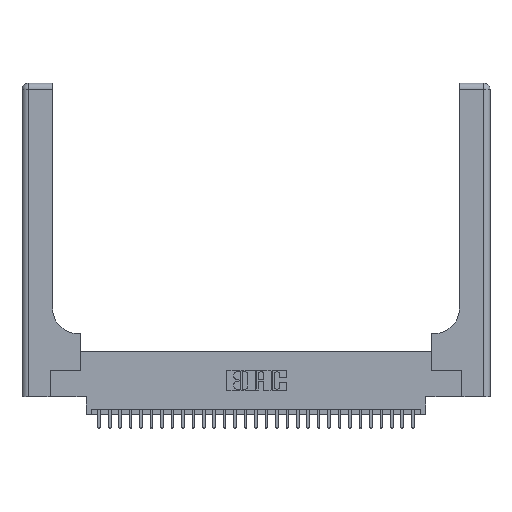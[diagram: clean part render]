
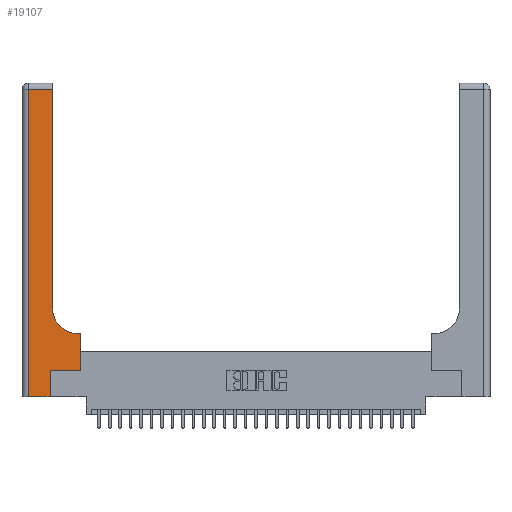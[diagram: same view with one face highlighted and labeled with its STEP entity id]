
A CAD part, top view. The second image highlights one B-rep face of the part: STEP entity #19107.
In plain terms, the highlighted planar face has unit normal (0, 0, 1).
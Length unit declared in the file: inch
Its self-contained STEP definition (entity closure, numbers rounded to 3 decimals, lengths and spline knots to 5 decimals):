
#305 = ORIENTED_EDGE ( 'NONE', *, *, #15811, .T. ) ;
#684 = VECTOR ( 'NONE', #5608, 39.37008 ) ;
#1043 = VERTEX_POINT ( 'NONE', #20322 ) ;
#1319 = DIRECTION ( 'NONE',  ( 1., 0., 0. ) ) ;
#2099 = EDGE_CURVE ( 'NONE', #4533, #7170, #13549, .T. ) ;
#2266 = ORIENTED_EDGE ( 'NONE', *, *, #24593, .T. ) ;
#2350 = CARTESIAN_POINT ( 'NONE',  ( 0.2915, 3., 0.37 ) ) ;
#2674 = VECTOR ( 'NONE', #5573, 39.37008 ) ;
#3101 = CARTESIAN_POINT ( 'NONE',  ( 0., 3., 0.37 ) ) ;
#3872 = VERTEX_POINT ( 'NONE', #9308 ) ;
#3947 = DIRECTION ( 'NONE',  ( 1., 0., 0. ) ) ;
#4533 = VERTEX_POINT ( 'NONE', #21021 ) ;
#4946 = LINE ( 'NONE', #23368, #9497 ) ;
#5573 = DIRECTION ( 'NONE',  ( 0., 1., 0. ) ) ;
#5608 = DIRECTION ( 'NONE',  ( 0., 1., 0. ) ) ;
#6122 = AXIS2_PLACEMENT_3D ( 'NONE', #3101, #25109, #22800 ) ;
#6243 = CARTESIAN_POINT ( 'NONE',  ( 0., 0., 0.37 ) ) ;
#6982 = CARTESIAN_POINT ( 'NONE',  ( 0.5415, 0.85, 0.37 ) ) ;
#7170 = VERTEX_POINT ( 'NONE', #9542 ) ;
#7971 = CARTESIAN_POINT ( 'NONE',  ( 0.5415, 0.6, 0.37 ) ) ;
#9214 = VERTEX_POINT ( 'NONE', #17256 ) ;
#9308 = CARTESIAN_POINT ( 'NONE',  ( 0.2915, 0.85, 0.37 ) ) ;
#9497 = VECTOR ( 'NONE', #28153, 39.37008 ) ;
#9542 = CARTESIAN_POINT ( 'NONE',  ( 0.269, 0.25, 0.37 ) ) ;
#10044 = EDGE_CURVE ( 'NONE', #7170, #30790, #30916, .T. ) ;
#10645 = VECTOR ( 'NONE', #1319, 39.37008 ) ;
#11177 = CARTESIAN_POINT ( 'NONE',  ( 0.5585, 0.6, 0.37 ) ) ;
#11581 = LINE ( 'NONE', #6243, #26584 ) ;
#13049 = VECTOR ( 'NONE', #29045, 39.37008 ) ;
#13188 = CARTESIAN_POINT ( 'NONE',  ( 0.269, 0., 0.37 ) ) ;
#13229 = VERTEX_POINT ( 'NONE', #7971 ) ;
#13549 = LINE ( 'NONE', #13188, #684 ) ;
#15126 = EDGE_CURVE ( 'NONE', #13229, #3872, #16676, .T. ) ;
#15198 = ORIENTED_EDGE ( 'NONE', *, *, #21528, .T. ) ;
#15236 = CARTESIAN_POINT ( 'NONE',  ( 0.2915, 2.94, 0.37 ) ) ;
#15411 = ORIENTED_EDGE ( 'NONE', *, *, #29080, .T. ) ;
#15711 = CARTESIAN_POINT ( 'NONE',  ( 0.5585, 0.25, 0.37 ) ) ;
#15811 = EDGE_CURVE ( 'NONE', #30790, #24294, #21904, .T. ) ;
#16215 = EDGE_CURVE ( 'NONE', #9214, #1043, #4946, .T. ) ;
#16245 = FACE_OUTER_BOUND ( 'NONE', #27070, .T. ) ;
#16252 = DIRECTION ( 'NONE',  ( 0., 0., -1. ) ) ;
#16676 = CIRCLE ( 'NONE', #16720, 0.25 ) ;
#16720 = AXIS2_PLACEMENT_3D ( 'NONE', #6982, #16252, #23535 ) ;
#16874 = ORIENTED_EDGE ( 'NONE', *, *, #15126, .T. ) ;
#17256 = CARTESIAN_POINT ( 'NONE',  ( 0.06, 2.94, 0.37 ) ) ;
#19107 = ADVANCED_FACE ( 'NONE', ( #16245 ), #24789, .F. ) ;
#20137 = ORIENTED_EDGE ( 'NONE', *, *, #16215, .T. ) ;
#20200 = LINE ( 'NONE', #2350, #13049 ) ;
#20322 = CARTESIAN_POINT ( 'NONE',  ( 0.06, 0., 0.37 ) ) ;
#20371 = EDGE_CURVE ( 'NONE', #28719, #9214, #24096, .T. ) ;
#20741 = ORIENTED_EDGE ( 'NONE', *, *, #2099, .T. ) ;
#21021 = CARTESIAN_POINT ( 'NONE',  ( 0.269, 0., 0.37 ) ) ;
#21222 = LINE ( 'NONE', #26559, #21957 ) ;
#21528 = EDGE_CURVE ( 'NONE', #1043, #4533, #11581, .T. ) ;
#21571 = DIRECTION ( 'NONE',  ( -1., 0., 0. ) ) ;
#21870 = DIRECTION ( 'NONE',  ( -1., 0., 0. ) ) ;
#21904 = LINE ( 'NONE', #28798, #2674 ) ;
#21957 = VECTOR ( 'NONE', #21870, 39.37008 ) ;
#22800 = DIRECTION ( 'NONE',  ( -1., 0., 0. ) ) ;
#23368 = CARTESIAN_POINT ( 'NONE',  ( 0.06, 3., 0.37 ) ) ;
#23427 = ORIENTED_EDGE ( 'NONE', *, *, #10044, .T. ) ;
#23535 = DIRECTION ( 'NONE',  ( 1., 0., 0. ) ) ;
#23589 = ORIENTED_EDGE ( 'NONE', *, *, #20371, .T. ) ;
#24096 = LINE ( 'NONE', #26273, #29706 ) ;
#24294 = VERTEX_POINT ( 'NONE', #11177 ) ;
#24593 = EDGE_CURVE ( 'NONE', #24294, #13229, #21222, .T. ) ;
#24789 = PLANE ( 'NONE',  #6122 ) ;
#24893 = CARTESIAN_POINT ( 'NONE',  ( 0.269, 0.25, 0.37 ) ) ;
#25109 = DIRECTION ( 'NONE',  ( 0., 0., -1. ) ) ;
#26273 = CARTESIAN_POINT ( 'NONE',  ( 0., 2.94, 0.37 ) ) ;
#26559 = CARTESIAN_POINT ( 'NONE',  ( 0.2915, 0.6, 0.37 ) ) ;
#26584 = VECTOR ( 'NONE', #3947, 39.37008 ) ;
#27070 = EDGE_LOOP ( 'NONE', ( #15411, #23589, #20137, #15198, #20741, #23427, #305, #2266, #16874 ) ) ;
#28153 = DIRECTION ( 'NONE',  ( 0., -1., 0. ) ) ;
#28719 = VERTEX_POINT ( 'NONE', #15236 ) ;
#28798 = CARTESIAN_POINT ( 'NONE',  ( 0.5585, 0.25, 0.37 ) ) ;
#29045 = DIRECTION ( 'NONE',  ( 0., 1., 0. ) ) ;
#29080 = EDGE_CURVE ( 'NONE', #3872, #28719, #20200, .T. ) ;
#29706 = VECTOR ( 'NONE', #21571, 39.37008 ) ;
#30790 = VERTEX_POINT ( 'NONE', #15711 ) ;
#30916 = LINE ( 'NONE', #24893, #10645 ) ;
